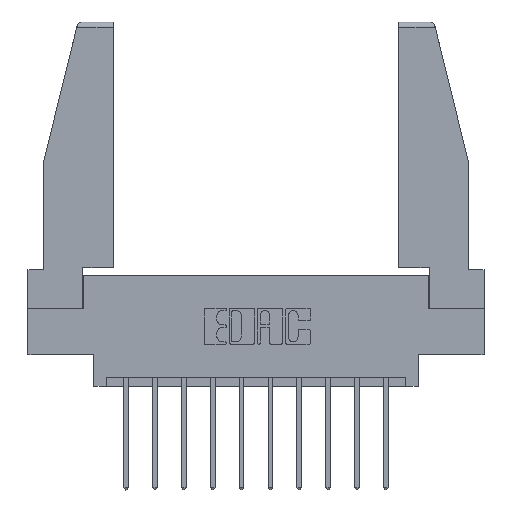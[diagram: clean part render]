
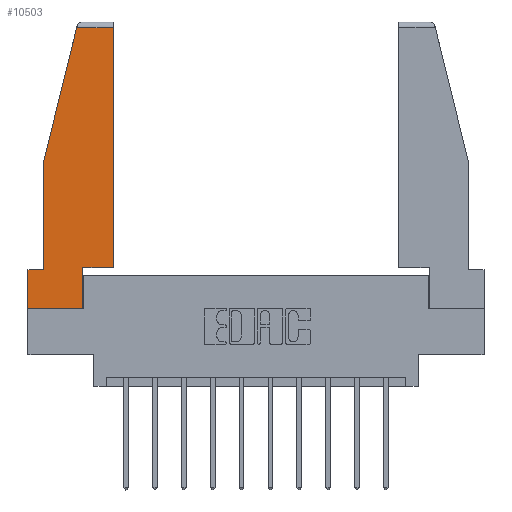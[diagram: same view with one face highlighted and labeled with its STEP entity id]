
A CAD part, top view. The second image highlights one B-rep face of the part: STEP entity #10503.
In plain terms, the highlighted planar face has unit normal (0, 0, 1).
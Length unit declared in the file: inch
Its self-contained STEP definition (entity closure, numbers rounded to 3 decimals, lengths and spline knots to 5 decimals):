
#146 = DIRECTION ( 'NONE',  ( -1., 0., 0. ) ) ;
#196 = EDGE_LOOP ( 'NONE', ( #10752, #8305, #8498, #10448, #1333, #8303, #8124, #329, #12507 ) ) ;
#325 = CARTESIAN_POINT ( 'NONE',  ( 0., 1.52, 0. ) ) ;
#329 = ORIENTED_EDGE ( 'NONE', *, *, #11099, .T. ) ;
#430 = VECTOR ( 'NONE', #2766, 39.37008 ) ;
#747 = CARTESIAN_POINT ( 'NONE',  ( 0.297, 0.223, 0. ) ) ;
#763 = EDGE_CURVE ( 'NONE', #5578, #1740, #13943, .T. ) ;
#1006 = AXIS2_PLACEMENT_3D ( 'NONE', #10997, #5385, #9929 ) ;
#1054 = VERTEX_POINT ( 'NONE', #3577 ) ;
#1260 = VECTOR ( 'NONE', #9711, 39.37008 ) ;
#1333 = ORIENTED_EDGE ( 'NONE', *, *, #5327, .T. ) ;
#1465 = LINE ( 'NONE', #10037, #13043 ) ;
#1488 = VECTOR ( 'NONE', #146, 39.37008 ) ;
#1630 = FACE_OUTER_BOUND ( 'NONE', #196, .T. ) ;
#1740 = VERTEX_POINT ( 'NONE', #6787 ) ;
#2426 = CARTESIAN_POINT ( 'NONE',  ( 0., 0.21, 0. ) ) ;
#2590 = VERTEX_POINT ( 'NONE', #4103 ) ;
#2736 = VERTEX_POINT ( 'NONE', #12844 ) ;
#2766 = DIRECTION ( 'NONE',  ( -0.239, -0.971, 0. ) ) ;
#3178 = DIRECTION ( 'NONE',  ( 0., -1., 0. ) ) ;
#3577 = CARTESIAN_POINT ( 'NONE',  ( 0.461, 0.223, 0. ) ) ;
#3702 = LINE ( 'NONE', #8630, #1260 ) ;
#4103 = CARTESIAN_POINT ( 'NONE',  ( 0.461, 1.52, 0. ) ) ;
#4178 = DIRECTION ( 'NONE',  ( 1., 0., 0. ) ) ;
#4587 = LINE ( 'NONE', #747, #13180 ) ;
#4593 = EDGE_CURVE ( 'NONE', #2590, #5578, #5189, .T. ) ;
#4836 = CARTESIAN_POINT ( 'NONE',  ( 0.297, 0.223, 0. ) ) ;
#5100 = CARTESIAN_POINT ( 'NONE',  ( 0., 0., 0. ) ) ;
#5189 = LINE ( 'NONE', #325, #1488 ) ;
#5309 = CARTESIAN_POINT ( 'NONE',  ( 0.086, 0.21, 0. ) ) ;
#5327 = EDGE_CURVE ( 'NONE', #6082, #12834, #10057, .T. ) ;
#5385 = DIRECTION ( 'NONE',  ( 0., 0., 1. ) ) ;
#5578 = VERTEX_POINT ( 'NONE', #10808 ) ;
#5824 = DIRECTION ( 'NONE',  ( 1., 0., 0. ) ) ;
#6082 = VERTEX_POINT ( 'NONE', #5309 ) ;
#6464 = PLANE ( 'NONE',  #1006 ) ;
#6475 = CARTESIAN_POINT ( 'NONE',  ( 0.086, 0.8, 0. ) ) ;
#6503 = EDGE_CURVE ( 'NONE', #12664, #2736, #10714, .T. ) ;
#6612 = CARTESIAN_POINT ( 'NONE',  ( 0., 0., 0. ) ) ;
#6787 = CARTESIAN_POINT ( 'NONE',  ( 0.086, 0.8, 0. ) ) ;
#6841 = EDGE_CURVE ( 'NONE', #7779, #1054, #4587, .T. ) ;
#7373 = CARTESIAN_POINT ( 'NONE',  ( 0.271, 1.55, 0. ) ) ;
#7779 = VERTEX_POINT ( 'NONE', #4836 ) ;
#8124 = ORIENTED_EDGE ( 'NONE', *, *, #6503, .T. ) ;
#8258 = LINE ( 'NONE', #13623, #10691 ) ;
#8303 = ORIENTED_EDGE ( 'NONE', *, *, #9305, .T. ) ;
#8305 = ORIENTED_EDGE ( 'NONE', *, *, #4593, .T. ) ;
#8498 = ORIENTED_EDGE ( 'NONE', *, *, #763, .T. ) ;
#8630 = CARTESIAN_POINT ( 'NONE',  ( 0.297, 0., 0. ) ) ;
#9305 = EDGE_CURVE ( 'NONE', #12834, #12664, #1465, .T. ) ;
#9701 = VECTOR ( 'NONE', #12361, 39.37008 ) ;
#9711 = DIRECTION ( 'NONE',  ( 0., 1., 0. ) ) ;
#9929 = DIRECTION ( 'NONE',  ( 1., 0., 0. ) ) ;
#10036 = VECTOR ( 'NONE', #14180, 39.37008 ) ;
#10037 = CARTESIAN_POINT ( 'NONE',  ( 0., 0.21, 0. ) ) ;
#10057 = LINE ( 'NONE', #2426, #9701 ) ;
#10324 = CARTESIAN_POINT ( 'NONE',  ( 0., 0.21, 0. ) ) ;
#10448 = ORIENTED_EDGE ( 'NONE', *, *, #13360, .T. ) ;
#10503 = ADVANCED_FACE ( 'NONE', ( #1630 ), #6464, .T. ) ;
#10691 = VECTOR ( 'NONE', #13761, 39.37008 ) ;
#10714 = LINE ( 'NONE', #6612, #13357 ) ;
#10752 = ORIENTED_EDGE ( 'NONE', *, *, #11434, .T. ) ;
#10808 = CARTESIAN_POINT ( 'NONE',  ( 0.2636, 1.52, 0. ) ) ;
#10997 = CARTESIAN_POINT ( 'NONE',  ( 0., 0., 0. ) ) ;
#11099 = EDGE_CURVE ( 'NONE', #2736, #7779, #3702, .T. ) ;
#11434 = EDGE_CURVE ( 'NONE', #1054, #2590, #8258, .T. ) ;
#12361 = DIRECTION ( 'NONE',  ( -1., 0., 0. ) ) ;
#12507 = ORIENTED_EDGE ( 'NONE', *, *, #6841, .T. ) ;
#12664 = VERTEX_POINT ( 'NONE', #5100 ) ;
#12834 = VERTEX_POINT ( 'NONE', #10324 ) ;
#12844 = CARTESIAN_POINT ( 'NONE',  ( 0.297, 0., 0. ) ) ;
#13043 = VECTOR ( 'NONE', #3178, 39.37008 ) ;
#13180 = VECTOR ( 'NONE', #4178, 39.37008 ) ;
#13357 = VECTOR ( 'NONE', #5824, 39.37008 ) ;
#13360 = EDGE_CURVE ( 'NONE', #1740, #6082, #13540, .T. ) ;
#13540 = LINE ( 'NONE', #6475, #10036 ) ;
#13623 = CARTESIAN_POINT ( 'NONE',  ( 0.461, 0.223, 0. ) ) ;
#13761 = DIRECTION ( 'NONE',  ( 0., 1., 0. ) ) ;
#13943 = LINE ( 'NONE', #7373, #430 ) ;
#14180 = DIRECTION ( 'NONE',  ( 0., -1., 0. ) ) ;
